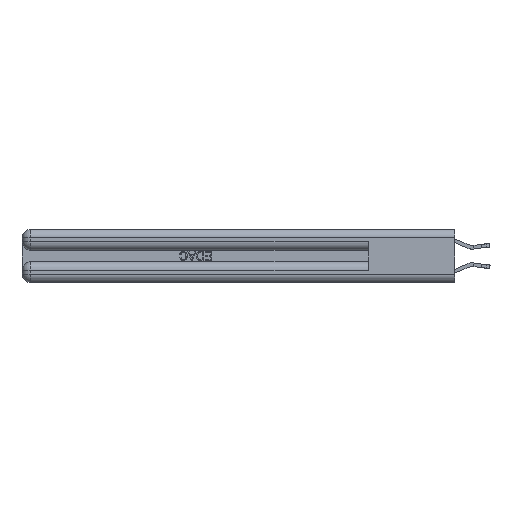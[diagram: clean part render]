
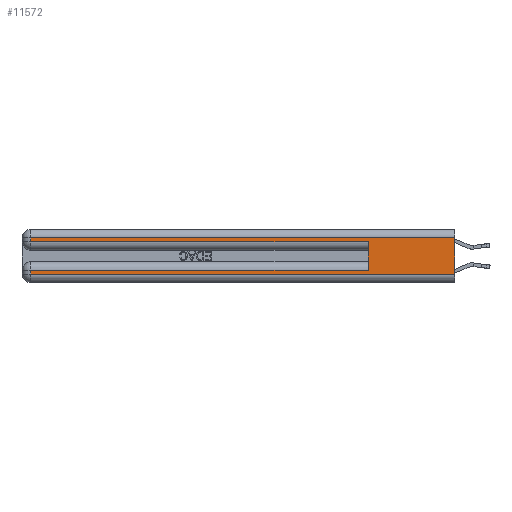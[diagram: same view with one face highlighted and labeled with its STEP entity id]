
A CAD part, left-side view. The second image highlights one B-rep face of the part: STEP entity #11572.
In plain terms, the highlighted planar face has unit normal (-1, 0, 0).
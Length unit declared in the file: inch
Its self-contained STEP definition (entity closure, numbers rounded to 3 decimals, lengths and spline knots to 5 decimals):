
#58 = CARTESIAN_POINT ( 'NONE',  ( 0., 2.94, 0.285 ) ) ;
#206 = CARTESIAN_POINT ( 'NONE',  ( 0., 2.94, 0.085 ) ) ;
#316 = ORIENTED_EDGE ( 'NONE', *, *, #20909, .F. ) ;
#1431 = VECTOR ( 'NONE', #24359, 39.37008 ) ;
#2230 = ORIENTED_EDGE ( 'NONE', *, *, #12657, .T. ) ;
#2599 = DIRECTION ( 'NONE',  ( 1., 0., 0. ) ) ;
#3214 = VECTOR ( 'NONE', #21293, 39.37008 ) ;
#3276 = EDGE_CURVE ( 'NONE', #8721, #5813, #17535, .T. ) ;
#3864 = CARTESIAN_POINT ( 'NONE',  ( 0., 0., 0.285 ) ) ;
#4175 = FACE_OUTER_BOUND ( 'NONE', #16367, .T. ) ;
#5813 = VERTEX_POINT ( 'NONE', #206 ) ;
#6215 = LINE ( 'NONE', #23573, #3214 ) ;
#6473 = DIRECTION ( 'NONE',  ( 0., -1., 0. ) ) ;
#7327 = LINE ( 'NONE', #14250, #24079 ) ;
#8456 = VERTEX_POINT ( 'NONE', #16594 ) ;
#8495 = LINE ( 'NONE', #28768, #30819 ) ;
#8721 = VERTEX_POINT ( 'NONE', #30366 ) ;
#8893 = VERTEX_POINT ( 'NONE', #17087 ) ;
#8904 = VECTOR ( 'NONE', #17268, 39.37008 ) ;
#9092 = ORIENTED_EDGE ( 'NONE', *, *, #3276, .T. ) ;
#10149 = CARTESIAN_POINT ( 'NONE',  ( 0., 0., 0.31 ) ) ;
#10194 = ORIENTED_EDGE ( 'NONE', *, *, #27310, .T. ) ;
#10372 = CARTESIAN_POINT ( 'NONE',  ( 0., 2.94, 0.31 ) ) ;
#11391 = DIRECTION ( 'NONE',  ( 0., 0., -1. ) ) ;
#11572 = ADVANCED_FACE ( 'NONE', ( #4175 ), #24181, .F. ) ;
#12034 = DIRECTION ( 'NONE',  ( 0., 0., -1. ) ) ;
#12361 = CARTESIAN_POINT ( 'NONE',  ( 0., 0., 0.37 ) ) ;
#12434 = LINE ( 'NONE', #27890, #18006 ) ;
#12657 = EDGE_CURVE ( 'NONE', #26422, #8893, #21996, .T. ) ;
#14250 = CARTESIAN_POINT ( 'NONE',  ( 0., 0.6, 0.145 ) ) ;
#15018 = EDGE_CURVE ( 'NONE', #19210, #21679, #6215, .T. ) ;
#16367 = EDGE_LOOP ( 'NONE', ( #29371, #25330, #24434, #16499, #316, #9092, #10194, #2230 ) ) ;
#16499 = ORIENTED_EDGE ( 'NONE', *, *, #30820, .T. ) ;
#16594 = CARTESIAN_POINT ( 'NONE',  ( 0., 0.6, 0.285 ) ) ;
#16610 = CARTESIAN_POINT ( 'NONE',  ( 0., 0., 0.085 ) ) ;
#16680 = EDGE_CURVE ( 'NONE', #21679, #22513, #12434, .T. ) ;
#17087 = CARTESIAN_POINT ( 'NONE',  ( 0., 0., 0.06 ) ) ;
#17268 = DIRECTION ( 'NONE',  ( 0., 1., 0. ) ) ;
#17535 = LINE ( 'NONE', #16610, #8904 ) ;
#17589 = LINE ( 'NONE', #3864, #20176 ) ;
#18006 = VECTOR ( 'NONE', #20893, 39.37008 ) ;
#19210 = VERTEX_POINT ( 'NONE', #10149 ) ;
#20169 = EDGE_CURVE ( 'NONE', #19210, #8893, #8495, .T. ) ;
#20176 = VECTOR ( 'NONE', #6473, 39.37008 ) ;
#20797 = LINE ( 'NONE', #20842, #24154 ) ;
#20842 = CARTESIAN_POINT ( 'NONE',  ( 0., 2.94, 0.37 ) ) ;
#20893 = DIRECTION ( 'NONE',  ( 0., 0., -1. ) ) ;
#20909 = EDGE_CURVE ( 'NONE', #8721, #8456, #7327, .T. ) ;
#21293 = DIRECTION ( 'NONE',  ( 0., 1., 0. ) ) ;
#21679 = VERTEX_POINT ( 'NONE', #10372 ) ;
#21996 = LINE ( 'NONE', #26788, #1431 ) ;
#22513 = VERTEX_POINT ( 'NONE', #58 ) ;
#23573 = CARTESIAN_POINT ( 'NONE',  ( 0., 0., 0.31 ) ) ;
#23662 = DIRECTION ( 'NONE',  ( 0., 0., -1. ) ) ;
#24079 = VECTOR ( 'NONE', #30860, 39.37008 ) ;
#24154 = VECTOR ( 'NONE', #11391, 39.37008 ) ;
#24181 = PLANE ( 'NONE',  #26742 ) ;
#24359 = DIRECTION ( 'NONE',  ( 0., -1., 0. ) ) ;
#24434 = ORIENTED_EDGE ( 'NONE', *, *, #16680, .T. ) ;
#25330 = ORIENTED_EDGE ( 'NONE', *, *, #15018, .T. ) ;
#26422 = VERTEX_POINT ( 'NONE', #29455 ) ;
#26742 = AXIS2_PLACEMENT_3D ( 'NONE', #12361, #2599, #12034 ) ;
#26788 = CARTESIAN_POINT ( 'NONE',  ( 0., 0., 0.06 ) ) ;
#27310 = EDGE_CURVE ( 'NONE', #5813, #26422, #20797, .T. ) ;
#27890 = CARTESIAN_POINT ( 'NONE',  ( 0., 2.94, 0.37 ) ) ;
#28768 = CARTESIAN_POINT ( 'NONE',  ( 0., 0., 0.37 ) ) ;
#29371 = ORIENTED_EDGE ( 'NONE', *, *, #20169, .F. ) ;
#29455 = CARTESIAN_POINT ( 'NONE',  ( 0., 2.94, 0.06 ) ) ;
#30366 = CARTESIAN_POINT ( 'NONE',  ( 0., 0.6, 0.085 ) ) ;
#30819 = VECTOR ( 'NONE', #23662, 39.37008 ) ;
#30820 = EDGE_CURVE ( 'NONE', #22513, #8456, #17589, .T. ) ;
#30860 = DIRECTION ( 'NONE',  ( 0., 0., 1. ) ) ;
